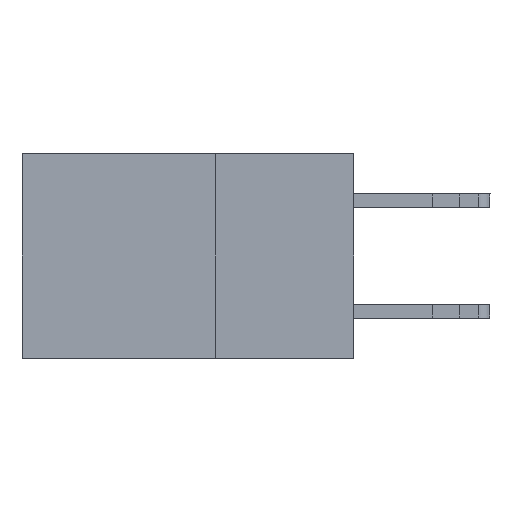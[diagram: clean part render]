
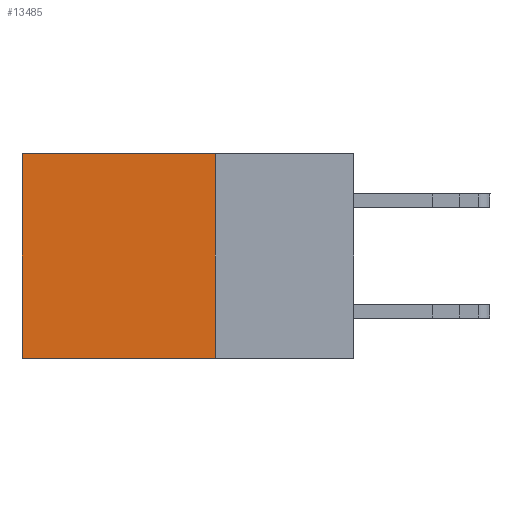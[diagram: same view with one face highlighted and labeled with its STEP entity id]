
A CAD part, left-side view. The second image highlights one B-rep face of the part: STEP entity #13485.
In plain terms, the highlighted planar face has unit normal (-1, 0, 0).
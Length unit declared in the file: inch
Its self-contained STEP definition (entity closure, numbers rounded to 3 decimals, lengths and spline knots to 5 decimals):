
#333 = CARTESIAN_POINT ( 'NONE',  ( 0.2875, 0.6, 0. ) ) ;
#439 = LINE ( 'NONE', #550, #2952 ) ;
#467 = DIRECTION ( 'NONE',  ( 0., 0., -1. ) ) ;
#550 = CARTESIAN_POINT ( 'NONE',  ( 0.2875, 0.25, -0.37 ) ) ;
#1044 = LINE ( 'NONE', #13274, #10676 ) ;
#1523 = VERTEX_POINT ( 'NONE', #333 ) ;
#2040 = VERTEX_POINT ( 'NONE', #20343 ) ;
#2952 = VECTOR ( 'NONE', #9370, 39.37008 ) ;
#4501 = DIRECTION ( 'NONE',  ( 0., 1., 0. ) ) ;
#4835 = DIRECTION ( 'NONE',  ( 0., 0., -1. ) ) ;
#5091 = ORIENTED_EDGE ( 'NONE', *, *, #21968, .F. ) ;
#5434 = AXIS2_PLACEMENT_3D ( 'NONE', #10113, #20688, #4835 ) ;
#6032 = CARTESIAN_POINT ( 'NONE',  ( 0.2875, 0.25, 0. ) ) ;
#6249 = LINE ( 'NONE', #6032, #16404 ) ;
#9059 = CARTESIAN_POINT ( 'NONE',  ( 0.2875, 0.25, 0. ) ) ;
#9370 = DIRECTION ( 'NONE',  ( 0., 1., 0. ) ) ;
#9439 = ORIENTED_EDGE ( 'NONE', *, *, #17620, .T. ) ;
#10113 = CARTESIAN_POINT ( 'NONE',  ( 0.2875, 0.25, 0. ) ) ;
#10676 = VECTOR ( 'NONE', #20225, 39.37008 ) ;
#11563 = ORIENTED_EDGE ( 'NONE', *, *, #20323, .T. ) ;
#13274 = CARTESIAN_POINT ( 'NONE',  ( 0.2875, 0.6, 0. ) ) ;
#13485 = ADVANCED_FACE ( 'NONE', ( #13748 ), #17152, .F. ) ;
#13748 = FACE_OUTER_BOUND ( 'NONE', #15944, .T. ) ;
#15944 = EDGE_LOOP ( 'NONE', ( #9439, #18941, #5091, #11563 ) ) ;
#16404 = VECTOR ( 'NONE', #4501, 39.37008 ) ;
#16466 = VECTOR ( 'NONE', #467, 39.37008 ) ;
#16646 = CARTESIAN_POINT ( 'NONE',  ( 0.2875, 0.6, -0.37 ) ) ;
#17152 = PLANE ( 'NONE',  #5434 ) ;
#17620 = EDGE_CURVE ( 'NONE', #1523, #17995, #1044, .T. ) ;
#17995 = VERTEX_POINT ( 'NONE', #16646 ) ;
#18941 = ORIENTED_EDGE ( 'NONE', *, *, #22406, .F. ) ;
#19795 = VERTEX_POINT ( 'NONE', #21209 ) ;
#20225 = DIRECTION ( 'NONE',  ( 0., 0., -1. ) ) ;
#20323 = EDGE_CURVE ( 'NONE', #19795, #1523, #6249, .T. ) ;
#20343 = CARTESIAN_POINT ( 'NONE',  ( 0.2875, 0.25, -0.37 ) ) ;
#20688 = DIRECTION ( 'NONE',  ( 1., 0., 0. ) ) ;
#21209 = CARTESIAN_POINT ( 'NONE',  ( 0.2875, 0.25, 0. ) ) ;
#21233 = LINE ( 'NONE', #9059, #16466 ) ;
#21968 = EDGE_CURVE ( 'NONE', #19795, #2040, #21233, .T. ) ;
#22406 = EDGE_CURVE ( 'NONE', #2040, #17995, #439, .T. ) ;
